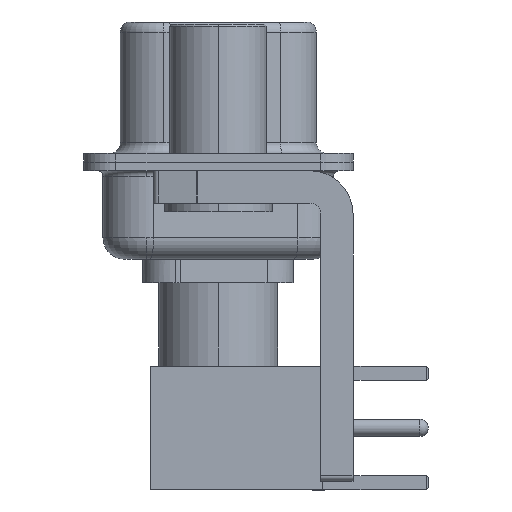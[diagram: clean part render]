
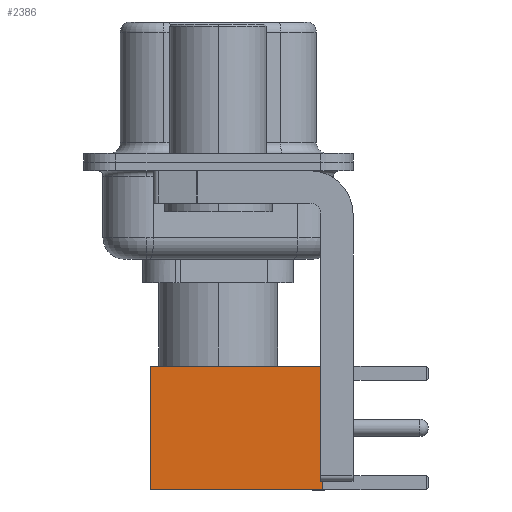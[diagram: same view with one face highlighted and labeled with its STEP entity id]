
A CAD part, left-side view. The second image highlights one B-rep face of the part: STEP entity #2386.
In plain terms, the highlighted face is planar.
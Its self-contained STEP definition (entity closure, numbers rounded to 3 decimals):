
#240 = VECTOR ( 'NONE', #674, 1000. ) ;
#383 = DIRECTION ( 'NONE',  ( 0., 1., 0. ) ) ;
#582 = CARTESIAN_POINT ( 'NONE',  ( 2.875, 2.875, 0. ) ) ;
#674 = DIRECTION ( 'NONE',  ( 0., 0., -1. ) ) ;
#1116 = EDGE_CURVE ( 'NONE', #9177, #18269, #5324, .T. ) ;
#2278 = EDGE_LOOP ( 'NONE', ( #18520, #11326, #14779, #10517 ) ) ;
#2386 = ADVANCED_FACE ( 'NONE', ( #3217 ), #4730, .T. ) ;
#2420 = DIRECTION ( 'NONE',  ( -1., 0., 0. ) ) ;
#2923 = VERTEX_POINT ( 'NONE', #9549 ) ;
#2941 = EDGE_CURVE ( 'NONE', #2923, #9177, #10978, .T. ) ;
#3217 = FACE_OUTER_BOUND ( 'NONE', #2278, .T. ) ;
#4435 = DIRECTION ( 'NONE',  ( 0., 0., -1. ) ) ;
#4730 = PLANE ( 'NONE',  #14315 ) ;
#5324 = LINE ( 'NONE', #11504, #240 ) ;
#5574 = CARTESIAN_POINT ( 'NONE',  ( 0., 2.875, 0. ) ) ;
#5656 = LINE ( 'NONE', #12230, #16174 ) ;
#6060 = CARTESIAN_POINT ( 'NONE',  ( -2.875, 2.875, 0. ) ) ;
#6967 = EDGE_CURVE ( 'NONE', #18426, #18269, #13466, .T. ) ;
#8293 = VECTOR ( 'NONE', #2420, 1000. ) ;
#9177 = VERTEX_POINT ( 'NONE', #15913 ) ;
#9549 = CARTESIAN_POINT ( 'NONE',  ( 2.875, 2.875, 8. ) ) ;
#10517 = ORIENTED_EDGE ( 'NONE', *, *, #2941, .F. ) ;
#10907 = CARTESIAN_POINT ( 'NONE',  ( 2.875, 2.875, 0. ) ) ;
#10978 = LINE ( 'NONE', #12501, #16911 ) ;
#11326 = ORIENTED_EDGE ( 'NONE', *, *, #6967, .T. ) ;
#11504 = CARTESIAN_POINT ( 'NONE',  ( -2.875, 2.875, 0. ) ) ;
#12230 = CARTESIAN_POINT ( 'NONE',  ( 2.875, 2.875, 0. ) ) ;
#12501 = CARTESIAN_POINT ( 'NONE',  ( 0., 2.875, 8. ) ) ;
#13466 = LINE ( 'NONE', #5574, #8293 ) ;
#14162 = EDGE_CURVE ( 'NONE', #2923, #18426, #5656, .T. ) ;
#14315 = AXIS2_PLACEMENT_3D ( 'NONE', #10907, #383, #15459 ) ;
#14779 = ORIENTED_EDGE ( 'NONE', *, *, #1116, .F. ) ;
#15459 = DIRECTION ( 'NONE',  ( 0., 0., 1. ) ) ;
#15730 = DIRECTION ( 'NONE',  ( -1., 0., 0. ) ) ;
#15913 = CARTESIAN_POINT ( 'NONE',  ( -2.875, 2.875, 8. ) ) ;
#16174 = VECTOR ( 'NONE', #4435, 1000. ) ;
#16911 = VECTOR ( 'NONE', #15730, 1000. ) ;
#18269 = VERTEX_POINT ( 'NONE', #6060 ) ;
#18426 = VERTEX_POINT ( 'NONE', #582 ) ;
#18520 = ORIENTED_EDGE ( 'NONE', *, *, #14162, .T. ) ;
